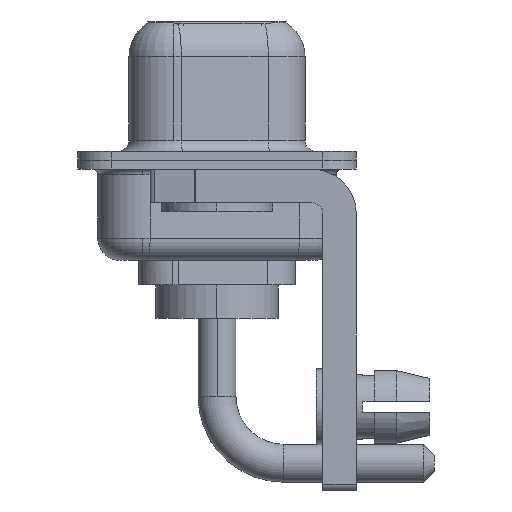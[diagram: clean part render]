
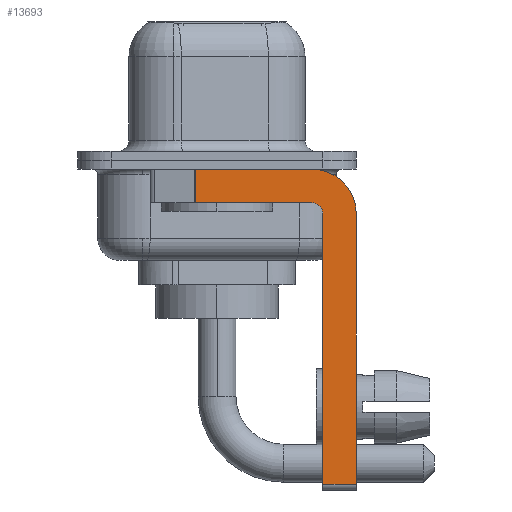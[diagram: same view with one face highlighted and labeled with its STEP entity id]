
A CAD part, left-side view. The second image highlights one B-rep face of the part: STEP entity #13693.
In plain terms, the highlighted planar face has unit normal (-1, 0, 0).
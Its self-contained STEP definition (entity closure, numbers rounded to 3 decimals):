
#83 = AXIS2_PLACEMENT_3D ( 'NONE', #2259, #4396, #13240 ) ;
#215 = FACE_OUTER_BOUND ( 'NONE', #7141, .T. ) ;
#424 = VERTEX_POINT ( 'NONE', #2292 ) ;
#688 = DIRECTION ( 'NONE',  ( 0., 0., -1. ) ) ;
#806 = VERTEX_POINT ( 'NONE', #13661 ) ;
#835 = EDGE_CURVE ( 'NONE', #3298, #424, #13521, .T. ) ;
#1588 = VECTOR ( 'NONE', #10432, 1000. ) ;
#2259 = CARTESIAN_POINT ( 'NONE',  ( -2.9, -4.25, -2.4 ) ) ;
#2286 = DIRECTION ( 'NONE',  ( 1., 0., 0. ) ) ;
#2292 = CARTESIAN_POINT ( 'NONE',  ( -2.9, 0.978, -1.9 ) ) ;
#2490 = LINE ( 'NONE', #2632, #7572 ) ;
#2632 = CARTESIAN_POINT ( 'NONE',  ( -2.9, 3., -0.4 ) ) ;
#2715 = EDGE_CURVE ( 'NONE', #10358, #3298, #8241, .T. ) ;
#2755 = LINE ( 'NONE', #3761, #13890 ) ;
#2784 = DIRECTION ( 'NONE',  ( 0., 0., 1. ) ) ;
#3298 = VERTEX_POINT ( 'NONE', #8832 ) ;
#3378 = CARTESIAN_POINT ( 'NONE',  ( -2.9, -4.25, -2.4 ) ) ;
#3587 = PLANE ( 'NONE',  #4132 ) ;
#3671 = VECTOR ( 'NONE', #11750, 1000. ) ;
#3724 = EDGE_CURVE ( 'NONE', #10767, #10358, #11695, .T. ) ;
#3756 = DIRECTION ( 'NONE',  ( 0., 0., 1. ) ) ;
#3761 = CARTESIAN_POINT ( 'NONE',  ( -2.9, 0.978, -1.9 ) ) ;
#3836 = CARTESIAN_POINT ( 'NONE',  ( -2.9, -4.25, -2.4 ) ) ;
#3838 = ORIENTED_EDGE ( 'NONE', *, *, #10824, .F. ) ;
#4132 = AXIS2_PLACEMENT_3D ( 'NONE', #3378, #2286, #10385 ) ;
#4237 = CARTESIAN_POINT ( 'NONE',  ( -2.9, -4.25, -0.4 ) ) ;
#4278 = DIRECTION ( 'NONE',  ( 0., 0., -1. ) ) ;
#4331 = VERTEX_POINT ( 'NONE', #4237 ) ;
#4364 = ORIENTED_EDGE ( 'NONE', *, *, #6285, .T. ) ;
#4396 = DIRECTION ( 'NONE',  ( 1., 0., 0. ) ) ;
#4688 = DIRECTION ( 'NONE',  ( 0., -1., 0. ) ) ;
#4907 = LINE ( 'NONE', #4977, #3671 ) ;
#4962 = AXIS2_PLACEMENT_3D ( 'NONE', #3836, #14008, #3756 ) ;
#4977 = CARTESIAN_POINT ( 'NONE',  ( -2.9, -4.25, -14.55 ) ) ;
#5245 = CARTESIAN_POINT ( 'NONE',  ( -2.9, -6.25, -2.4 ) ) ;
#5611 = ORIENTED_EDGE ( 'NONE', *, *, #3724, .F. ) ;
#5935 = CARTESIAN_POINT ( 'NONE',  ( -2.9, -4.25, -1.9 ) ) ;
#6285 = EDGE_CURVE ( 'NONE', #10615, #424, #2755, .T. ) ;
#6609 = CARTESIAN_POINT ( 'NONE',  ( -2.9, -4.75, -14.55 ) ) ;
#6693 = CARTESIAN_POINT ( 'NONE',  ( -2.9, 0.978, -0.4 ) ) ;
#7141 = EDGE_LOOP ( 'NONE', ( #13326, #4364, #14260, #10916, #5611, #11416, #8026, #3838 ) ) ;
#7393 = VERTEX_POINT ( 'NONE', #8804 ) ;
#7572 = VECTOR ( 'NONE', #4688, 1000. ) ;
#8010 = EDGE_CURVE ( 'NONE', #10615, #4331, #2490, .T. ) ;
#8026 = ORIENTED_EDGE ( 'NONE', *, *, #9799, .F. ) ;
#8241 = CIRCLE ( 'NONE', #4962, 0.5 ) ;
#8804 = CARTESIAN_POINT ( 'NONE',  ( -2.9, -6.25, -2.4 ) ) ;
#8832 = CARTESIAN_POINT ( 'NONE',  ( -2.9, -4.25, -1.9 ) ) ;
#9799 = EDGE_CURVE ( 'NONE', #7393, #806, #10848, .T. ) ;
#10122 = VECTOR ( 'NONE', #2784, 1000. ) ;
#10358 = VERTEX_POINT ( 'NONE', #14466 ) ;
#10385 = DIRECTION ( 'NONE',  ( 0., 0., -1. ) ) ;
#10432 = DIRECTION ( 'NONE',  ( 0., 1., 0. ) ) ;
#10615 = VERTEX_POINT ( 'NONE', #6693 ) ;
#10671 = CARTESIAN_POINT ( 'NONE',  ( -2.9, -4.75, -14.8 ) ) ;
#10767 = VERTEX_POINT ( 'NONE', #6609 ) ;
#10824 = EDGE_CURVE ( 'NONE', #4331, #7393, #12775, .T. ) ;
#10848 = LINE ( 'NONE', #5245, #14163 ) ;
#10916 = ORIENTED_EDGE ( 'NONE', *, *, #2715, .F. ) ;
#11416 = ORIENTED_EDGE ( 'NONE', *, *, #14208, .T. ) ;
#11695 = LINE ( 'NONE', #10671, #10122 ) ;
#11750 = DIRECTION ( 'NONE',  ( 0., -1., 0. ) ) ;
#12775 = CIRCLE ( 'NONE', #83, 2. ) ;
#13240 = DIRECTION ( 'NONE',  ( 0., 0., -1. ) ) ;
#13326 = ORIENTED_EDGE ( 'NONE', *, *, #8010, .F. ) ;
#13521 = LINE ( 'NONE', #5935, #1588 ) ;
#13661 = CARTESIAN_POINT ( 'NONE',  ( -2.9, -6.25, -14.55 ) ) ;
#13693 = ADVANCED_FACE ( 'NONE', ( #215 ), #3587, .F. ) ;
#13890 = VECTOR ( 'NONE', #688, 1000. ) ;
#14008 = DIRECTION ( 'NONE',  ( -1., 0., 0. ) ) ;
#14163 = VECTOR ( 'NONE', #4278, 1000. ) ;
#14208 = EDGE_CURVE ( 'NONE', #10767, #806, #4907, .T. ) ;
#14260 = ORIENTED_EDGE ( 'NONE', *, *, #835, .F. ) ;
#14466 = CARTESIAN_POINT ( 'NONE',  ( -2.9, -4.75, -2.4 ) ) ;
